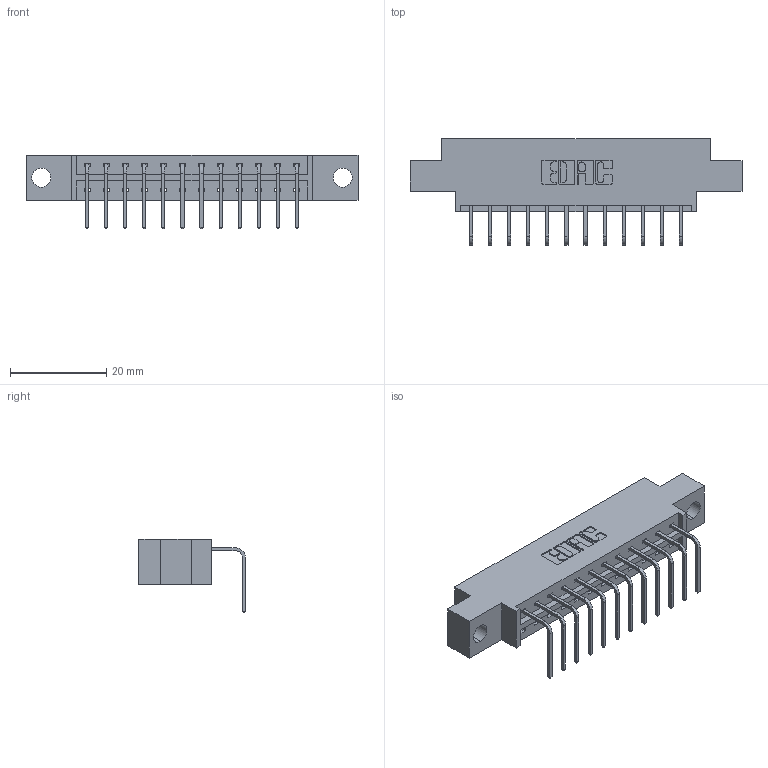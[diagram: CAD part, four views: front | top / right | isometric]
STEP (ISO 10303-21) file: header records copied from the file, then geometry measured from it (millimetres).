
FILE_DESCRIPTION (( 'STEP AP203' ), '1' );
FILE_NAME ('333-012-558-604.STEP', '2018-08-01T00:52:46', ( '' ), ( '' ), 'SwSTEP 2.0', 'SolidWorks 2016', '' );
FILE_SCHEMA (( 'CONFIG_CONTROL_DESIGN' ));
Length unit declared in the file: inch
Products named in the file (3): 333 Part_Offset - .156 Dia - TH; 345-292-001_558 Tail - 2; 333-012-558-604
Assembly tree (13 placements, depth 2):
  333-012-558-604
    333 Part_Offset - .156 Dia - TH
    345-292-001_558 Tail - 2  x12
Bounding box: 69.09 x 22.17 x 15.37 mm (x, y, z)
Volume: 6418.5 mm3; surface area: 6986.9 mm2
Topology: 13 solids, 13 shells, 838 faces, 2507 edges, 1654 vertices
Faces by surface type: plane 602, cylinder 236
Entity records: 11435 total; most frequent: CARTESIAN_POINT 1986, ORIENTED_EDGE 1934, DIRECTION 1735, EDGE_CURVE 967, LINE 839, VECTOR 839, VERTEX_POINT 642, AXIS2_PLACEMENT_3D 448
